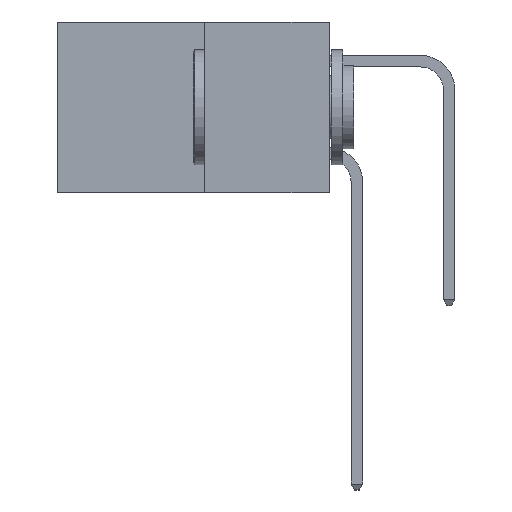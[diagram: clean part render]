
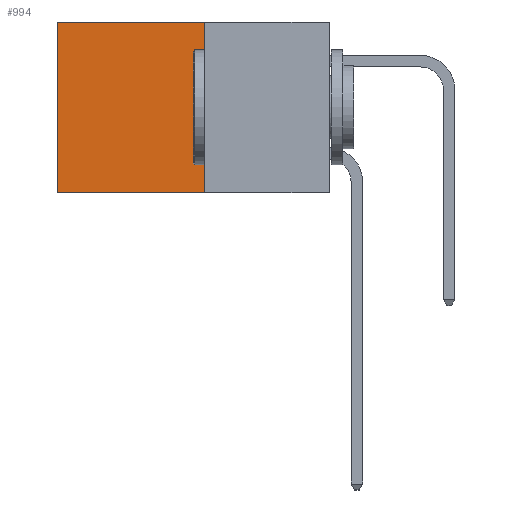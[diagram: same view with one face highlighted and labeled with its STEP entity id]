
A CAD part, left-side view. The second image highlights one B-rep face of the part: STEP entity #994.
In plain terms, the highlighted planar face has unit normal (-1, 0, 0).
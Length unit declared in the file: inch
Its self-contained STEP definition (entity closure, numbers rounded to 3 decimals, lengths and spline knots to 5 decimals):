
#173 = CARTESIAN_POINT ( 'NONE',  ( 0.277, 0.27, 0. ) ) ;
#509 = LINE ( 'NONE', #9320, #7567 ) ;
#706 = VERTEX_POINT ( 'NONE', #8321 ) ;
#818 = DIRECTION ( 'NONE',  ( 0., 1., 0. ) ) ;
#994 = ADVANCED_FACE ( 'NONE', ( #8915 ), #12094, .F. ) ;
#1089 = CARTESIAN_POINT ( 'NONE',  ( 0.277, 0.27, 0. ) ) ;
#2433 = VERTEX_POINT ( 'NONE', #173 ) ;
#2479 = VERTEX_POINT ( 'NONE', #9865 ) ;
#2886 = ORIENTED_EDGE ( 'NONE', *, *, #6046, .T. ) ;
#2981 = ORIENTED_EDGE ( 'NONE', *, *, #4848, .F. ) ;
#3257 = VECTOR ( 'NONE', #11345, 39.37008 ) ;
#3269 = LINE ( 'NONE', #1089, #12134 ) ;
#3772 = EDGE_LOOP ( 'NONE', ( #2886, #11629, #2981, #12102 ) ) ;
#4349 = EDGE_CURVE ( 'NONE', #2433, #706, #3269, .T. ) ;
#4848 = EDGE_CURVE ( 'NONE', #2433, #5580, #5049, .T. ) ;
#5049 = LINE ( 'NONE', #8994, #10294 ) ;
#5580 = VERTEX_POINT ( 'NONE', #11384 ) ;
#5582 = EDGE_CURVE ( 'NONE', #5580, #2479, #5771, .T. ) ;
#5771 = LINE ( 'NONE', #11457, #3257 ) ;
#6046 = EDGE_CURVE ( 'NONE', #706, #2479, #509, .T. ) ;
#7567 = VECTOR ( 'NONE', #9297, 39.37008 ) ;
#8321 = CARTESIAN_POINT ( 'NONE',  ( 0.277, 0.59, 0. ) ) ;
#8764 = DIRECTION ( 'NONE',  ( 0., 0., -1. ) ) ;
#8915 = FACE_OUTER_BOUND ( 'NONE', #3772, .T. ) ;
#8994 = CARTESIAN_POINT ( 'NONE',  ( 0.277, 0.27, -0.37 ) ) ;
#9124 = AXIS2_PLACEMENT_3D ( 'NONE', #11186, #10724, #11175 ) ;
#9297 = DIRECTION ( 'NONE',  ( 0., 0., -1. ) ) ;
#9320 = CARTESIAN_POINT ( 'NONE',  ( 0.277, 0.59, -0.37 ) ) ;
#9865 = CARTESIAN_POINT ( 'NONE',  ( 0.277, 0.59, -0.37 ) ) ;
#10294 = VECTOR ( 'NONE', #8764, 39.37008 ) ;
#10724 = DIRECTION ( 'NONE',  ( 1., 0., 0. ) ) ;
#11175 = DIRECTION ( 'NONE',  ( 0., 0., -1. ) ) ;
#11186 = CARTESIAN_POINT ( 'NONE',  ( 0.277, 0.27, -0.37 ) ) ;
#11345 = DIRECTION ( 'NONE',  ( 0., 1., 0. ) ) ;
#11384 = CARTESIAN_POINT ( 'NONE',  ( 0.277, 0.27, -0.37 ) ) ;
#11457 = CARTESIAN_POINT ( 'NONE',  ( 0.277, 0.27, -0.37 ) ) ;
#11629 = ORIENTED_EDGE ( 'NONE', *, *, #5582, .F. ) ;
#12094 = PLANE ( 'NONE',  #9124 ) ;
#12102 = ORIENTED_EDGE ( 'NONE', *, *, #4349, .T. ) ;
#12134 = VECTOR ( 'NONE', #818, 39.37008 ) ;
